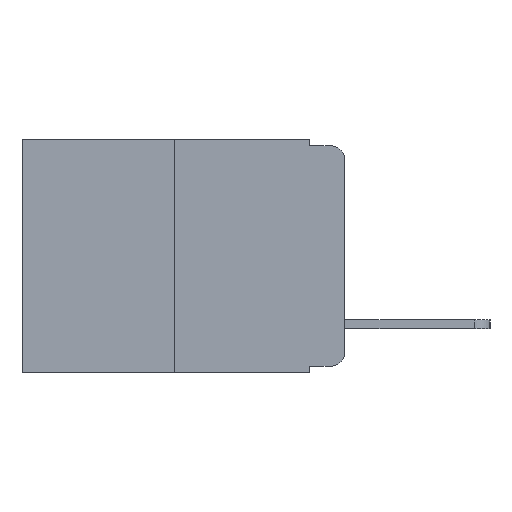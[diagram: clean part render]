
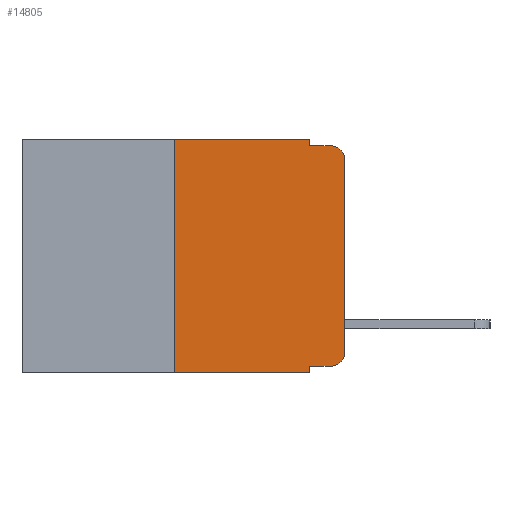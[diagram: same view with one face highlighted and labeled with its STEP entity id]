
A CAD part, left-side view. The second image highlights one B-rep face of the part: STEP entity #14805.
In plain terms, the highlighted planar face has unit normal (-1, 0, 0).
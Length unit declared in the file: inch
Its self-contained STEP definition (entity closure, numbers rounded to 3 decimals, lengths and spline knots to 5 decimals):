
#377 = VERTEX_POINT ( 'NONE', #8006 ) ;
#468 = DIRECTION ( 'NONE',  ( 0., 0., -1. ) ) ;
#593 = DIRECTION ( 'NONE',  ( 0., -1., 0. ) ) ;
#969 = DIRECTION ( 'NONE',  ( 0., -1., 0. ) ) ;
#1572 = CARTESIAN_POINT ( 'NONE',  ( 0., 0.051, -0.01 ) ) ;
#2156 = LINE ( 'NONE', #9539, #15305 ) ;
#2697 = DIRECTION ( 'NONE',  ( 0., 0., 1. ) ) ;
#3189 = CARTESIAN_POINT ( 'NONE',  ( 0., 0.051, -0.343 ) ) ;
#3362 = VECTOR ( 'NONE', #20526, 39.37008 ) ;
#3737 = VECTOR ( 'NONE', #468, 39.37008 ) ;
#3954 = ORIENTED_EDGE ( 'NONE', *, *, #12847, .F. ) ;
#4120 = VERTEX_POINT ( 'NONE', #15286 ) ;
#4262 = LINE ( 'NONE', #11459, #21528 ) ;
#4307 = LINE ( 'NONE', #14388, #3737 ) ;
#4346 = PLANE ( 'NONE',  #9059 ) ;
#4942 = CARTESIAN_POINT ( 'NONE',  ( 0., 0.02, -0.01 ) ) ;
#5026 = EDGE_CURVE ( 'NONE', #14779, #377, #8150, .T. ) ;
#5281 = CARTESIAN_POINT ( 'NONE',  ( 0., 0.02, -0.03 ) ) ;
#6098 = LINE ( 'NONE', #12914, #6631 ) ;
#6147 = EDGE_CURVE ( 'NONE', #4120, #13887, #19527, .T. ) ;
#6482 = DIRECTION ( 'NONE',  ( 0., 0., -1. ) ) ;
#6575 = ORIENTED_EDGE ( 'NONE', *, *, #6147, .T. ) ;
#6631 = VECTOR ( 'NONE', #2697, 39.37008 ) ;
#6725 = CARTESIAN_POINT ( 'NONE',  ( 0., 0., -0.313 ) ) ;
#7007 = DIRECTION ( 'NONE',  ( 0., 0., -1. ) ) ;
#7111 = VERTEX_POINT ( 'NONE', #4942 ) ;
#7229 = CARTESIAN_POINT ( 'NONE',  ( 0., 0.25, 0. ) ) ;
#7332 = EDGE_CURVE ( 'NONE', #9614, #4120, #7550, .T. ) ;
#7360 = CARTESIAN_POINT ( 'NONE',  ( 0., 0.02, -0.313 ) ) ;
#7550 = LINE ( 'NONE', #9061, #10895 ) ;
#7852 = DIRECTION ( 'NONE',  ( 0., 0., -1. ) ) ;
#8006 = CARTESIAN_POINT ( 'NONE',  ( 0., 0.051, 0. ) ) ;
#8150 = LINE ( 'NONE', #18643, #10959 ) ;
#8474 = EDGE_CURVE ( 'NONE', #9614, #10481, #15328, .T. ) ;
#8861 = ORIENTED_EDGE ( 'NONE', *, *, #8474, .F. ) ;
#8939 = CARTESIAN_POINT ( 'NONE',  ( 0., 0.051, -0.333 ) ) ;
#9025 = EDGE_LOOP ( 'NONE', ( #19234, #11392, #3954, #12928, #9104, #16139, #21521, #8861, #18252, #6575 ) ) ;
#9046 = EDGE_CURVE ( 'NONE', #10696, #10481, #2156, .T. ) ;
#9058 = DIRECTION ( 'NONE',  ( 0., 0., -1. ) ) ;
#9059 = AXIS2_PLACEMENT_3D ( 'NONE', #16152, #17853, #7852 ) ;
#9061 = CARTESIAN_POINT ( 'NONE',  ( 0., 0.051, -0.333 ) ) ;
#9104 = ORIENTED_EDGE ( 'NONE', *, *, #5026, .F. ) ;
#9539 = CARTESIAN_POINT ( 'NONE',  ( 0., 0.473, -0.343 ) ) ;
#9587 = EDGE_CURVE ( 'NONE', #10696, #14779, #21229, .T. ) ;
#9614 = VERTEX_POINT ( 'NONE', #8939 ) ;
#9911 = CARTESIAN_POINT ( 'NONE',  ( 0., 0.051, 0. ) ) ;
#10481 = VERTEX_POINT ( 'NONE', #3189 ) ;
#10696 = VERTEX_POINT ( 'NONE', #15425 ) ;
#10895 = VECTOR ( 'NONE', #17388, 39.37008 ) ;
#10959 = VECTOR ( 'NONE', #15316, 39.37008 ) ;
#11392 = ORIENTED_EDGE ( 'NONE', *, *, #15126, .T. ) ;
#11459 = CARTESIAN_POINT ( 'NONE',  ( 0., 0.051, -0.01 ) ) ;
#11765 = EDGE_CURVE ( 'NONE', #377, #19985, #4307, .T. ) ;
#11916 = VECTOR ( 'NONE', #6482, 39.37008 ) ;
#11931 = AXIS2_PLACEMENT_3D ( 'NONE', #5281, #17057, #7007 ) ;
#12847 = EDGE_CURVE ( 'NONE', #19985, #7111, #4262, .T. ) ;
#12914 = CARTESIAN_POINT ( 'NONE',  ( 0., 0., 0. ) ) ;
#12928 = ORIENTED_EDGE ( 'NONE', *, *, #11765, .F. ) ;
#13887 = VERTEX_POINT ( 'NONE', #6725 ) ;
#14388 = CARTESIAN_POINT ( 'NONE',  ( 0., 0.051, 0. ) ) ;
#14779 = VERTEX_POINT ( 'NONE', #17837 ) ;
#14805 = ADVANCED_FACE ( 'NONE', ( #18976 ), #4346, .F. ) ;
#15126 = EDGE_CURVE ( 'NONE', #19545, #7111, #20969, .T. ) ;
#15286 = CARTESIAN_POINT ( 'NONE',  ( 0., 0.02, -0.333 ) ) ;
#15305 = VECTOR ( 'NONE', #593, 39.37008 ) ;
#15316 = DIRECTION ( 'NONE',  ( 0., -1., 0. ) ) ;
#15328 = LINE ( 'NONE', #9911, #11916 ) ;
#15425 = CARTESIAN_POINT ( 'NONE',  ( 0., 0.25, -0.343 ) ) ;
#16139 = ORIENTED_EDGE ( 'NONE', *, *, #9587, .F. ) ;
#16152 = CARTESIAN_POINT ( 'NONE',  ( 0., 0.473, 0. ) ) ;
#16294 = EDGE_CURVE ( 'NONE', #13887, #19545, #6098, .T. ) ;
#17057 = DIRECTION ( 'NONE',  ( -1., 0., 0. ) ) ;
#17388 = DIRECTION ( 'NONE',  ( 0., -1., 0. ) ) ;
#17837 = CARTESIAN_POINT ( 'NONE',  ( 0., 0.25, 0. ) ) ;
#17853 = DIRECTION ( 'NONE',  ( 1., 0., 0. ) ) ;
#18252 = ORIENTED_EDGE ( 'NONE', *, *, #7332, .T. ) ;
#18643 = CARTESIAN_POINT ( 'NONE',  ( 0., 0.473, 0. ) ) ;
#18976 = FACE_OUTER_BOUND ( 'NONE', #9025, .T. ) ;
#19019 = DIRECTION ( 'NONE',  ( -1., 0., 0. ) ) ;
#19234 = ORIENTED_EDGE ( 'NONE', *, *, #16294, .T. ) ;
#19527 = CIRCLE ( 'NONE', #21945, 0.02 ) ;
#19545 = VERTEX_POINT ( 'NONE', #21224 ) ;
#19985 = VERTEX_POINT ( 'NONE', #1572 ) ;
#20526 = DIRECTION ( 'NONE',  ( 0., 0., 1. ) ) ;
#20969 = CIRCLE ( 'NONE', #11931, 0.02 ) ;
#21224 = CARTESIAN_POINT ( 'NONE',  ( 0., 0., -0.03 ) ) ;
#21229 = LINE ( 'NONE', #7229, #3362 ) ;
#21521 = ORIENTED_EDGE ( 'NONE', *, *, #9046, .T. ) ;
#21528 = VECTOR ( 'NONE', #969, 39.37008 ) ;
#21945 = AXIS2_PLACEMENT_3D ( 'NONE', #7360, #19019, #9058 ) ;
